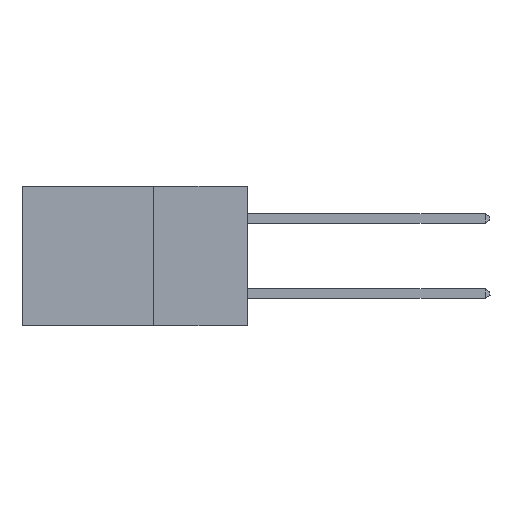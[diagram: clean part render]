
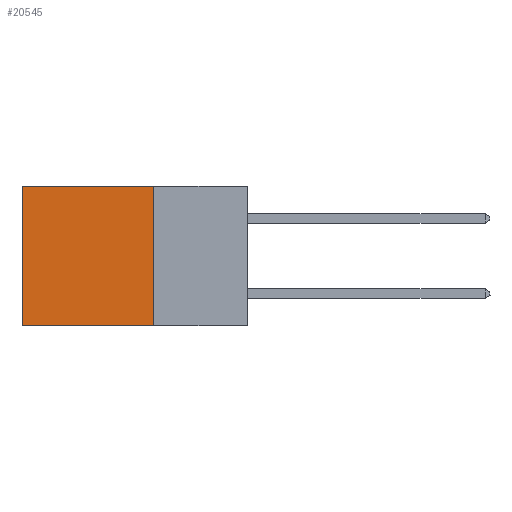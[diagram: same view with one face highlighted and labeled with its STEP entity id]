
A CAD part, left-side view. The second image highlights one B-rep face of the part: STEP entity #20545.
In plain terms, the highlighted planar face has unit normal (-1, 0, 0).
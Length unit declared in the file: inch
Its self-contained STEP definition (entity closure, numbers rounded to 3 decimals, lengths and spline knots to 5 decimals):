
#20 = DIRECTION ( 'NONE',  ( 0., 0., -1. ) ) ;
#292 = VECTOR ( 'NONE', #1534, 39.37008 ) ;
#1121 = VERTEX_POINT ( 'NONE', #17904 ) ;
#1534 = DIRECTION ( 'NONE',  ( 0., 1., 0. ) ) ;
#1866 = CARTESIAN_POINT ( 'NONE',  ( 0.298, 0.25, -0.37 ) ) ;
#3557 = EDGE_CURVE ( 'NONE', #1121, #10362, #13863, .T. ) ;
#3746 = CARTESIAN_POINT ( 'NONE',  ( 0.298, 0.6, 0. ) ) ;
#4939 = VERTEX_POINT ( 'NONE', #1866 ) ;
#5345 = DIRECTION ( 'NONE',  ( 0., 0., -1. ) ) ;
#5424 = EDGE_CURVE ( 'NONE', #14831, #4939, #19460, .T. ) ;
#5488 = LINE ( 'NONE', #24496, #292 ) ;
#5842 = CARTESIAN_POINT ( 'NONE',  ( 0.298, 0.25, 0. ) ) ;
#6460 = ORIENTED_EDGE ( 'NONE', *, *, #17886, .F. ) ;
#7342 = CARTESIAN_POINT ( 'NONE',  ( 0.298, 0.25, 0. ) ) ;
#7516 = VECTOR ( 'NONE', #20144, 39.37008 ) ;
#7947 = AXIS2_PLACEMENT_3D ( 'NONE', #5842, #11647, #20 ) ;
#8820 = VECTOR ( 'NONE', #5345, 39.37008 ) ;
#9032 = CARTESIAN_POINT ( 'NONE',  ( 0.298, 0.25, 0. ) ) ;
#10362 = VERTEX_POINT ( 'NONE', #18126 ) ;
#10691 = EDGE_LOOP ( 'NONE', ( #22162, #6460, #24353, #13904 ) ) ;
#11647 = DIRECTION ( 'NONE',  ( 1., 0., 0. ) ) ;
#12303 = FACE_OUTER_BOUND ( 'NONE', #10691, .T. ) ;
#13863 = LINE ( 'NONE', #3746, #8820 ) ;
#13904 = ORIENTED_EDGE ( 'NONE', *, *, #19218, .T. ) ;
#14831 = VERTEX_POINT ( 'NONE', #9032 ) ;
#17886 = EDGE_CURVE ( 'NONE', #4939, #10362, #5488, .T. ) ;
#17904 = CARTESIAN_POINT ( 'NONE',  ( 0.298, 0.6, 0. ) ) ;
#18126 = CARTESIAN_POINT ( 'NONE',  ( 0.298, 0.6, -0.37 ) ) ;
#18455 = VECTOR ( 'NONE', #22627, 39.37008 ) ;
#19218 = EDGE_CURVE ( 'NONE', #14831, #1121, #20419, .T. ) ;
#19460 = LINE ( 'NONE', #23468, #7516 ) ;
#20144 = DIRECTION ( 'NONE',  ( 0., 0., -1. ) ) ;
#20419 = LINE ( 'NONE', #7342, #18455 ) ;
#20545 = ADVANCED_FACE ( 'NONE', ( #12303 ), #23056, .F. ) ;
#22162 = ORIENTED_EDGE ( 'NONE', *, *, #3557, .T. ) ;
#22627 = DIRECTION ( 'NONE',  ( 0., 1., 0. ) ) ;
#23056 = PLANE ( 'NONE',  #7947 ) ;
#23468 = CARTESIAN_POINT ( 'NONE',  ( 0.298, 0.25, 0. ) ) ;
#24353 = ORIENTED_EDGE ( 'NONE', *, *, #5424, .F. ) ;
#24496 = CARTESIAN_POINT ( 'NONE',  ( 0.298, 0.25, -0.37 ) ) ;
